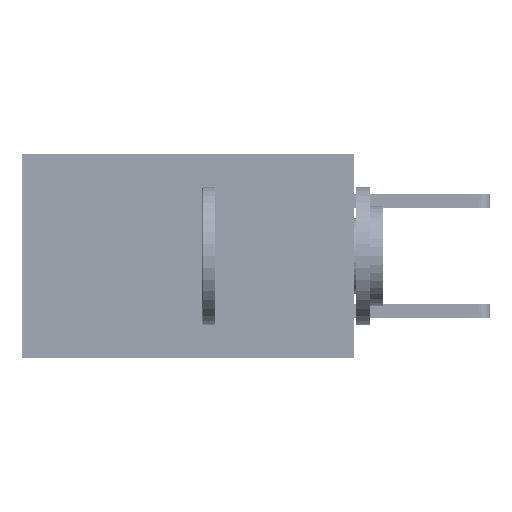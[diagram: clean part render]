
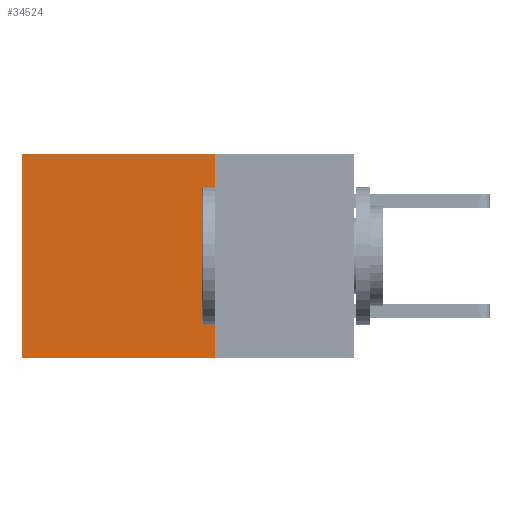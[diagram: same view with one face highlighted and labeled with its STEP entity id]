
A CAD part, left-side view. The second image highlights one B-rep face of the part: STEP entity #34524.
In plain terms, the highlighted planar face has unit normal (-1, 0, 0).
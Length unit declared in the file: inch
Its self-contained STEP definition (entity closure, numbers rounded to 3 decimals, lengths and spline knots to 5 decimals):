
#2538 = LINE ( 'NONE', #35554, #25929 ) ;
#3451 = DIRECTION ( 'NONE',  ( 0., 0., -1. ) ) ;
#4900 = EDGE_CURVE ( 'NONE', #29701, #9942, #2538, .T. ) ;
#5432 = EDGE_CURVE ( 'NONE', #26650, #21713, #45273, .T. ) ;
#5853 = CARTESIAN_POINT ( 'NONE',  ( 0.2875, 0.25, 0. ) ) ;
#8694 = DIRECTION ( 'NONE',  ( 0., 0., -1. ) ) ;
#9942 = VERTEX_POINT ( 'NONE', #41514 ) ;
#9964 = DIRECTION ( 'NONE',  ( 0., 0., -1. ) ) ;
#10639 = DIRECTION ( 'NONE',  ( 0., 1., 0. ) ) ;
#11673 = EDGE_CURVE ( 'NONE', #9942, #21713, #34817, .T. ) ;
#12392 = ORIENTED_EDGE ( 'NONE', *, *, #5432, .T. ) ;
#12565 = VECTOR ( 'NONE', #10639, 39.37008 ) ;
#14153 = CARTESIAN_POINT ( 'NONE',  ( 0.2875, 0.25, 0. ) ) ;
#17506 = PLANE ( 'NONE',  #38931 ) ;
#20870 = ORIENTED_EDGE ( 'NONE', *, *, #11673, .F. ) ;
#21713 = VERTEX_POINT ( 'NONE', #26125 ) ;
#23433 = LINE ( 'NONE', #27891, #38530 ) ;
#24348 = EDGE_LOOP ( 'NONE', ( #12392, #20870, #36525, #27563 ) ) ;
#25671 = CARTESIAN_POINT ( 'NONE',  ( 0.2875, 0.6, 0. ) ) ;
#25929 = VECTOR ( 'NONE', #8694, 39.37008 ) ;
#26125 = CARTESIAN_POINT ( 'NONE',  ( 0.2875, 0.6, -0.37 ) ) ;
#26650 = VERTEX_POINT ( 'NONE', #25671 ) ;
#27563 = ORIENTED_EDGE ( 'NONE', *, *, #31246, .T. ) ;
#27891 = CARTESIAN_POINT ( 'NONE',  ( 0.2875, 0.25, 0. ) ) ;
#29701 = VERTEX_POINT ( 'NONE', #5853 ) ;
#31246 = EDGE_CURVE ( 'NONE', #29701, #26650, #23433, .T. ) ;
#32596 = VECTOR ( 'NONE', #3451, 39.37008 ) ;
#33451 = FACE_OUTER_BOUND ( 'NONE', #24348, .T. ) ;
#34524 = ADVANCED_FACE ( 'NONE', ( #33451 ), #17506, .F. ) ;
#34817 = LINE ( 'NONE', #41265, #12565 ) ;
#35554 = CARTESIAN_POINT ( 'NONE',  ( 0.2875, 0.25, 0. ) ) ;
#36525 = ORIENTED_EDGE ( 'NONE', *, *, #4900, .F. ) ;
#38530 = VECTOR ( 'NONE', #43372, 39.37008 ) ;
#38931 = AXIS2_PLACEMENT_3D ( 'NONE', #14153, #44935, #9964 ) ;
#41265 = CARTESIAN_POINT ( 'NONE',  ( 0.2875, 0.25, -0.37 ) ) ;
#41514 = CARTESIAN_POINT ( 'NONE',  ( 0.2875, 0.25, -0.37 ) ) ;
#43372 = DIRECTION ( 'NONE',  ( 0., 1., 0. ) ) ;
#44935 = DIRECTION ( 'NONE',  ( 1., 0., 0. ) ) ;
#45273 = LINE ( 'NONE', #49509, #32596 ) ;
#49509 = CARTESIAN_POINT ( 'NONE',  ( 0.2875, 0.6, 0. ) ) ;
